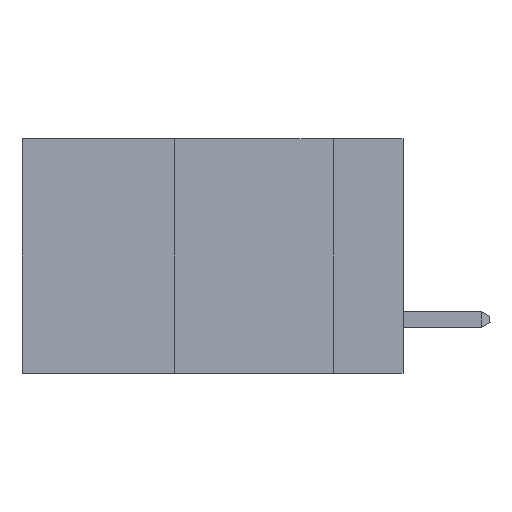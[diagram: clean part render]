
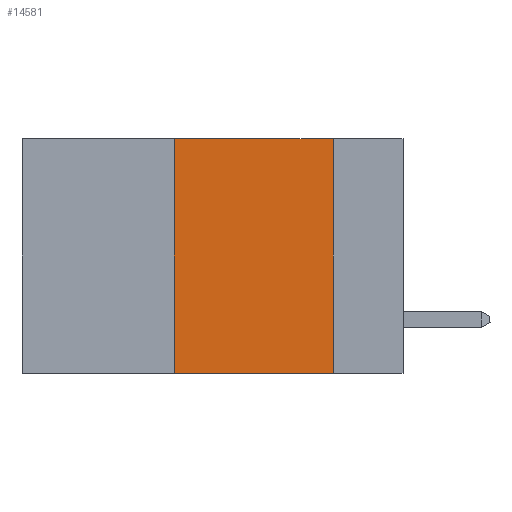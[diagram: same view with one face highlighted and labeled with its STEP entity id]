
A CAD part, left-side view. The second image highlights one B-rep face of the part: STEP entity #14581.
In plain terms, the highlighted planar face has unit normal (-1, 0, 0).
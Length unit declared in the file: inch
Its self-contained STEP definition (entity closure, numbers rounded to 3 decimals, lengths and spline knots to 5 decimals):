
#488 = LINE ( 'NONE', #7440, #1104 ) ;
#838 = EDGE_CURVE ( 'NONE', #14750, #11297, #18905, .T. ) ;
#1104 = VECTOR ( 'NONE', #16998, 39.37008 ) ;
#1797 = DIRECTION ( 'NONE',  ( 0., 0., -1. ) ) ;
#2401 = EDGE_CURVE ( 'NONE', #24504, #14750, #16947, .T. ) ;
#2444 = EDGE_LOOP ( 'NONE', ( #6522, #10755, #17257, #14658 ) ) ;
#3263 = CARTESIAN_POINT ( 'NONE',  ( 0., 0.11, -0.37 ) ) ;
#3504 = EDGE_CURVE ( 'NONE', #24504, #24617, #488, .T. ) ;
#5108 = CARTESIAN_POINT ( 'NONE',  ( 0., 0.6, 0. ) ) ;
#6522 = ORIENTED_EDGE ( 'NONE', *, *, #21604, .F. ) ;
#7047 = DIRECTION ( 'NONE',  ( 1., 0., 0. ) ) ;
#7440 = CARTESIAN_POINT ( 'NONE',  ( 0., 0.6, -0.37 ) ) ;
#8786 = CARTESIAN_POINT ( 'NONE',  ( 0., 0.6, 0. ) ) ;
#8980 = PLANE ( 'NONE',  #16159 ) ;
#10567 = CARTESIAN_POINT ( 'NONE',  ( 0., 0.36, -0.37 ) ) ;
#10755 = ORIENTED_EDGE ( 'NONE', *, *, #838, .F. ) ;
#11297 = VERTEX_POINT ( 'NONE', #17022 ) ;
#12087 = VECTOR ( 'NONE', #1797, 39.37008 ) ;
#13185 = CARTESIAN_POINT ( 'NONE',  ( 0., 0.36, 0. ) ) ;
#13332 = LINE ( 'NONE', #13595, #12087 ) ;
#13595 = CARTESIAN_POINT ( 'NONE',  ( 0., 0.11, 0. ) ) ;
#14581 = ADVANCED_FACE ( 'NONE', ( #16072 ), #8980, .F. ) ;
#14658 = ORIENTED_EDGE ( 'NONE', *, *, #3504, .T. ) ;
#14750 = VERTEX_POINT ( 'NONE', #13185 ) ;
#16072 = FACE_OUTER_BOUND ( 'NONE', #2444, .T. ) ;
#16159 = AXIS2_PLACEMENT_3D ( 'NONE', #5108, #7047, #20654 ) ;
#16320 = VECTOR ( 'NONE', #18752, 39.37008 ) ;
#16947 = LINE ( 'NONE', #20650, #16320 ) ;
#16998 = DIRECTION ( 'NONE',  ( 0., -1., 0. ) ) ;
#17022 = CARTESIAN_POINT ( 'NONE',  ( 0., 0.11, 0. ) ) ;
#17257 = ORIENTED_EDGE ( 'NONE', *, *, #2401, .F. ) ;
#18752 = DIRECTION ( 'NONE',  ( 0., 0., 1. ) ) ;
#18813 = DIRECTION ( 'NONE',  ( 0., -1., 0. ) ) ;
#18905 = LINE ( 'NONE', #8786, #25335 ) ;
#20650 = CARTESIAN_POINT ( 'NONE',  ( 0., 0.36, 0. ) ) ;
#20654 = DIRECTION ( 'NONE',  ( 0., 0., -1. ) ) ;
#21604 = EDGE_CURVE ( 'NONE', #11297, #24617, #13332, .T. ) ;
#24504 = VERTEX_POINT ( 'NONE', #10567 ) ;
#24617 = VERTEX_POINT ( 'NONE', #3263 ) ;
#25335 = VECTOR ( 'NONE', #18813, 39.37008 ) ;
